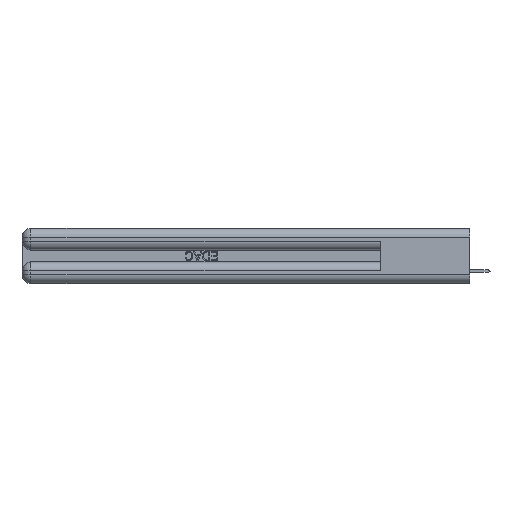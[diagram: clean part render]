
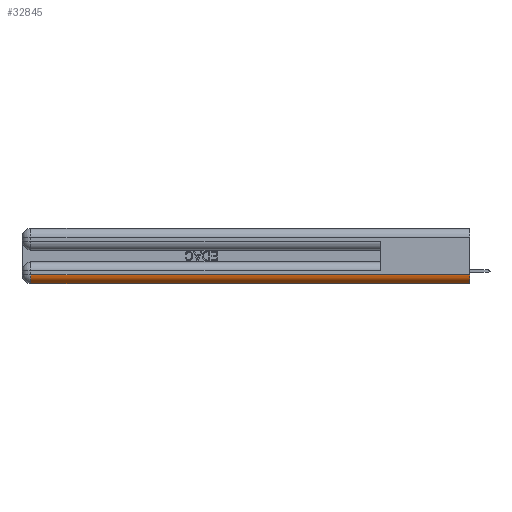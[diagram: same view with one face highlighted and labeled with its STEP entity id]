
A CAD part, left-side view. The second image highlights one B-rep face of the part: STEP entity #32845.
In plain terms, the highlighted cylindrical face has radius 1.524 mm (diameter 3.048 mm), a partial arc.
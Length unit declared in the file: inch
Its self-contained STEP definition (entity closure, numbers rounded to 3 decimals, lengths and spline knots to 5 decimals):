
#4846 = DIRECTION ( 'NONE',  ( 0., 0., 1. ) ) ;
#7419 = ORIENTED_EDGE ( 'NONE', *, *, #10326, .F. ) ;
#8664 = EDGE_CURVE ( 'NONE', #20779, #12440, #48447, .T. ) ;
#8864 = AXIS2_PLACEMENT_3D ( 'NONE', #12879, #16821, #48498 ) ;
#10326 = EDGE_CURVE ( 'NONE', #17407, #49928, #50697, .T. ) ;
#10812 = FACE_OUTER_BOUND ( 'NONE', #34115, .T. ) ;
#11079 = DIRECTION ( 'NONE',  ( 0., 1., 0. ) ) ;
#12440 = VERTEX_POINT ( 'NONE', #29018 ) ;
#12879 = CARTESIAN_POINT ( 'NONE',  ( 0.06, 2.94, 0.06 ) ) ;
#14710 = CARTESIAN_POINT ( 'NONE',  ( 0., 2.94, 0.06 ) ) ;
#14828 = VECTOR ( 'NONE', #35979, 39.37008 ) ;
#16821 = DIRECTION ( 'NONE',  ( 0., 1., 0. ) ) ;
#17217 = LINE ( 'NONE', #44751, #39642 ) ;
#17407 = VERTEX_POINT ( 'NONE', #31412 ) ;
#18376 = AXIS2_PLACEMENT_3D ( 'NONE', #20818, #32834, #4846 ) ;
#18934 = CYLINDRICAL_SURFACE ( 'NONE', #37892, 0.06 ) ;
#19429 = ORIENTED_EDGE ( 'NONE', *, *, #46063, .F. ) ;
#19968 = CARTESIAN_POINT ( 'NONE',  ( 0.06, 0., 0.06 ) ) ;
#20778 = ORIENTED_EDGE ( 'NONE', *, *, #40151, .F. ) ;
#20779 = VERTEX_POINT ( 'NONE', #24698 ) ;
#20818 = CARTESIAN_POINT ( 'NONE',  ( 0.06, 0., 0.06 ) ) ;
#23163 = LINE ( 'NONE', #39149, #14828 ) ;
#24698 = CARTESIAN_POINT ( 'NONE',  ( 0., 0., 0.06 ) ) ;
#29018 = CARTESIAN_POINT ( 'NONE',  ( 0.06, 0., 0. ) ) ;
#31412 = CARTESIAN_POINT ( 'NONE',  ( 0.06, 2.94, 0. ) ) ;
#32834 = DIRECTION ( 'NONE',  ( 0., -1., 0. ) ) ;
#32845 = ADVANCED_FACE ( 'NONE', ( #10812 ), #18934, .T. ) ;
#34115 = EDGE_LOOP ( 'NONE', ( #38605, #20778, #7419, #19429 ) ) ;
#35979 = DIRECTION ( 'NONE',  ( 0., 1., 0. ) ) ;
#37892 = AXIS2_PLACEMENT_3D ( 'NONE', #19968, #11079, #42799 ) ;
#38605 = ORIENTED_EDGE ( 'NONE', *, *, #8664, .F. ) ;
#39149 = CARTESIAN_POINT ( 'NONE',  ( 0.06, 3., 0. ) ) ;
#39642 = VECTOR ( 'NONE', #41078, 39.37008 ) ;
#40151 = EDGE_CURVE ( 'NONE', #49928, #20779, #17217, .T. ) ;
#41078 = DIRECTION ( 'NONE',  ( 0., -1., 0. ) ) ;
#42799 = DIRECTION ( 'NONE',  ( 0., 0., 1. ) ) ;
#44751 = CARTESIAN_POINT ( 'NONE',  ( 0., 0., 0.06 ) ) ;
#46063 = EDGE_CURVE ( 'NONE', #12440, #17407, #23163, .T. ) ;
#48447 = CIRCLE ( 'NONE', #18376, 0.06 ) ;
#48498 = DIRECTION ( 'NONE',  ( 0., 0., 1. ) ) ;
#49928 = VERTEX_POINT ( 'NONE', #14710 ) ;
#50697 = CIRCLE ( 'NONE', #8864, 0.06 ) ;
